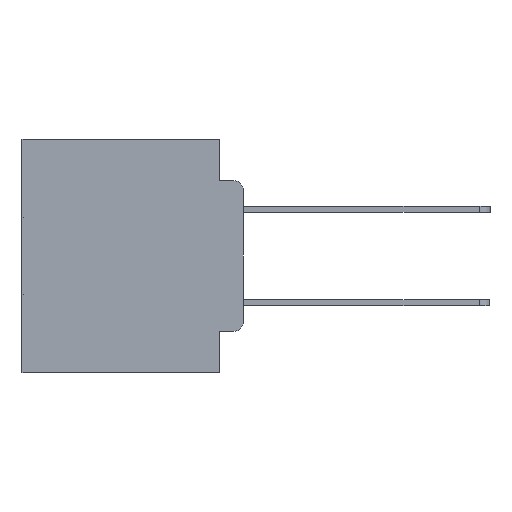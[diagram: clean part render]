
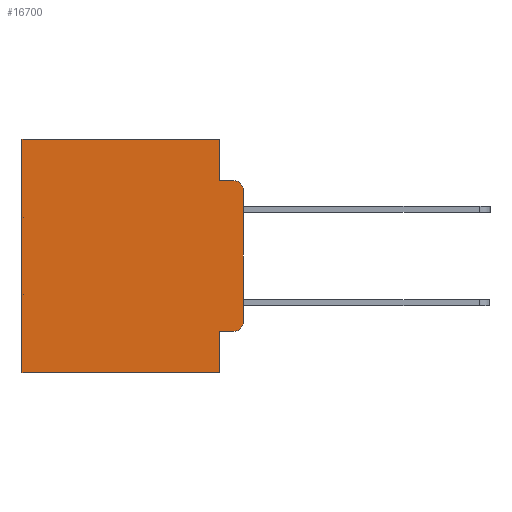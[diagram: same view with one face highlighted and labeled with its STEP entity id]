
A CAD part, left-side view. The second image highlights one B-rep face of the part: STEP entity #16700.
In plain terms, the highlighted planar face has unit normal (-1, 0, 0).
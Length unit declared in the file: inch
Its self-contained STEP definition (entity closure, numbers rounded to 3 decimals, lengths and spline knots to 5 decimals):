
#233 = EDGE_CURVE ( 'NONE', #5705, #19589, #7470, .T. ) ;
#268 = DIRECTION ( 'NONE',  ( 0., 0., -1. ) ) ;
#689 = EDGE_CURVE ( 'NONE', #4767, #29139, #2436, .T. ) ;
#1721 = ORIENTED_EDGE ( 'NONE', *, *, #30374, .T. ) ;
#1761 = EDGE_LOOP ( 'NONE', ( #13972, #3768, #24879, #20023, #7737, #28787, #10325, #11092, #1721, #20638 ) ) ;
#1964 = EDGE_CURVE ( 'NONE', #29139, #22866, #30540, .T. ) ;
#2416 = DIRECTION ( 'NONE',  ( 0., 0., -1. ) ) ;
#2436 = LINE ( 'NONE', #22952, #14928 ) ;
#3642 = VECTOR ( 'NONE', #21283, 39.37008 ) ;
#3768 = ORIENTED_EDGE ( 'NONE', *, *, #13774, .T. ) ;
#3810 = CARTESIAN_POINT ( 'NONE',  ( 0.298, 0.051, -0.5 ) ) ;
#4006 = CARTESIAN_POINT ( 'NONE',  ( 0.298, 0., 0. ) ) ;
#4425 = DIRECTION ( 'NONE',  ( 1., 0., 0. ) ) ;
#4767 = VERTEX_POINT ( 'NONE', #19035 ) ;
#5705 = VERTEX_POINT ( 'NONE', #17317 ) ;
#6573 = VERTEX_POINT ( 'NONE', #16067 ) ;
#7075 = EDGE_CURVE ( 'NONE', #4767, #30130, #21771, .T. ) ;
#7283 = DIRECTION ( 'NONE',  ( 0., 0., -1. ) ) ;
#7367 = FACE_OUTER_BOUND ( 'NONE', #1761, .T. ) ;
#7470 = LINE ( 'NONE', #30181, #26845 ) ;
#7656 = LINE ( 'NONE', #22389, #19944 ) ;
#7737 = ORIENTED_EDGE ( 'NONE', *, *, #689, .T. ) ;
#9107 = AXIS2_PLACEMENT_3D ( 'NONE', #21586, #4425, #21697 ) ;
#9398 = VECTOR ( 'NONE', #19196, 39.37008 ) ;
#10325 = ORIENTED_EDGE ( 'NONE', *, *, #12543, .F. ) ;
#11092 = ORIENTED_EDGE ( 'NONE', *, *, #233, .F. ) ;
#11160 = VERTEX_POINT ( 'NONE', #20450 ) ;
#12117 = EDGE_CURVE ( 'NONE', #30130, #11160, #31123, .T. ) ;
#12543 = EDGE_CURVE ( 'NONE', #19589, #22866, #7656, .T. ) ;
#13352 = DIRECTION ( 'NONE',  ( -1., 0., 0. ) ) ;
#13397 = CIRCLE ( 'NONE', #29934, 0.02 ) ;
#13411 = DIRECTION ( 'NONE',  ( 0., -1., 0. ) ) ;
#13586 = CIRCLE ( 'NONE', #31065, 0.02 ) ;
#13774 = EDGE_CURVE ( 'NONE', #16181, #11160, #13397, .T. ) ;
#13972 = ORIENTED_EDGE ( 'NONE', *, *, #28209, .F. ) ;
#14928 = VECTOR ( 'NONE', #28854, 39.37008 ) ;
#15290 = DIRECTION ( 'NONE',  ( -1., 0., 0. ) ) ;
#16067 = CARTESIAN_POINT ( 'NONE',  ( 0.298, 0., -0.3915 ) ) ;
#16181 = VERTEX_POINT ( 'NONE', #24430 ) ;
#16681 = LINE ( 'NONE', #19096, #9398 ) ;
#16700 = ADVANCED_FACE ( 'NONE', ( #7367 ), #16790, .F. ) ;
#16790 = PLANE ( 'NONE',  #9107 ) ;
#17317 = CARTESIAN_POINT ( 'NONE',  ( 0.298, 0.051, -0.4115 ) ) ;
#17368 = DIRECTION ( 'NONE',  ( 0., 1., 0. ) ) ;
#17860 = VECTOR ( 'NONE', #7283, 39.37008 ) ;
#19035 = CARTESIAN_POINT ( 'NONE',  ( 0.298, 0.051, 0. ) ) ;
#19096 = CARTESIAN_POINT ( 'NONE',  ( 0.298, 0.051, -0.4115 ) ) ;
#19196 = DIRECTION ( 'NONE',  ( 0., -1., 0. ) ) ;
#19589 = VERTEX_POINT ( 'NONE', #3810 ) ;
#19944 = VECTOR ( 'NONE', #17368, 39.37008 ) ;
#20023 = ORIENTED_EDGE ( 'NONE', *, *, #7075, .F. ) ;
#20450 = CARTESIAN_POINT ( 'NONE',  ( 0.298, 0.02, -0.0885 ) ) ;
#20638 = ORIENTED_EDGE ( 'NONE', *, *, #25621, .T. ) ;
#21012 = VECTOR ( 'NONE', #27544, 39.37008 ) ;
#21283 = DIRECTION ( 'NONE',  ( 0., 0., -1. ) ) ;
#21509 = CARTESIAN_POINT ( 'NONE',  ( 0.298, 0.02, -0.4115 ) ) ;
#21586 = CARTESIAN_POINT ( 'NONE',  ( 0.298, 0., 0. ) ) ;
#21634 = CARTESIAN_POINT ( 'NONE',  ( 0.298, 0.473, -0.5 ) ) ;
#21697 = DIRECTION ( 'NONE',  ( 0., 0., -1. ) ) ;
#21771 = LINE ( 'NONE', #30337, #21012 ) ;
#22389 = CARTESIAN_POINT ( 'NONE',  ( 0.298, 0., -0.5 ) ) ;
#22866 = VERTEX_POINT ( 'NONE', #21634 ) ;
#22952 = CARTESIAN_POINT ( 'NONE',  ( 0.298, 0., 0. ) ) ;
#23125 = CARTESIAN_POINT ( 'NONE',  ( 0.298, 0.051, -0.0885 ) ) ;
#23300 = LINE ( 'NONE', #4006, #3642 ) ;
#23500 = VERTEX_POINT ( 'NONE', #21509 ) ;
#24430 = CARTESIAN_POINT ( 'NONE',  ( 0.298, 0., -0.1085 ) ) ;
#24879 = ORIENTED_EDGE ( 'NONE', *, *, #12117, .F. ) ;
#25558 = VECTOR ( 'NONE', #13411, 39.37008 ) ;
#25621 = EDGE_CURVE ( 'NONE', #23500, #6573, #13586, .T. ) ;
#26845 = VECTOR ( 'NONE', #2416, 39.37008 ) ;
#27544 = DIRECTION ( 'NONE',  ( 0., 0., -1. ) ) ;
#27705 = CARTESIAN_POINT ( 'NONE',  ( 0.298, 0.02, -0.3915 ) ) ;
#27870 = CARTESIAN_POINT ( 'NONE',  ( 0.298, 0.051, -0.0885 ) ) ;
#28209 = EDGE_CURVE ( 'NONE', #16181, #6573, #23300, .T. ) ;
#28628 = CARTESIAN_POINT ( 'NONE',  ( 0.298, 0.473, 0. ) ) ;
#28787 = ORIENTED_EDGE ( 'NONE', *, *, #1964, .T. ) ;
#28854 = DIRECTION ( 'NONE',  ( 0., 1., 0. ) ) ;
#29139 = VERTEX_POINT ( 'NONE', #28628 ) ;
#29619 = CARTESIAN_POINT ( 'NONE',  ( 0.298, 0.02, -0.1085 ) ) ;
#29934 = AXIS2_PLACEMENT_3D ( 'NONE', #29619, #15290, #268 ) ;
#30080 = DIRECTION ( 'NONE',  ( 0., 0., -1. ) ) ;
#30130 = VERTEX_POINT ( 'NONE', #27870 ) ;
#30181 = CARTESIAN_POINT ( 'NONE',  ( 0.298, 0.051, 0. ) ) ;
#30255 = CARTESIAN_POINT ( 'NONE',  ( 0.298, 0.473, 0. ) ) ;
#30337 = CARTESIAN_POINT ( 'NONE',  ( 0.298, 0.051, 0. ) ) ;
#30374 = EDGE_CURVE ( 'NONE', #5705, #23500, #16681, .T. ) ;
#30540 = LINE ( 'NONE', #30255, #17860 ) ;
#31065 = AXIS2_PLACEMENT_3D ( 'NONE', #27705, #13352, #30080 ) ;
#31123 = LINE ( 'NONE', #23125, #25558 ) ;
